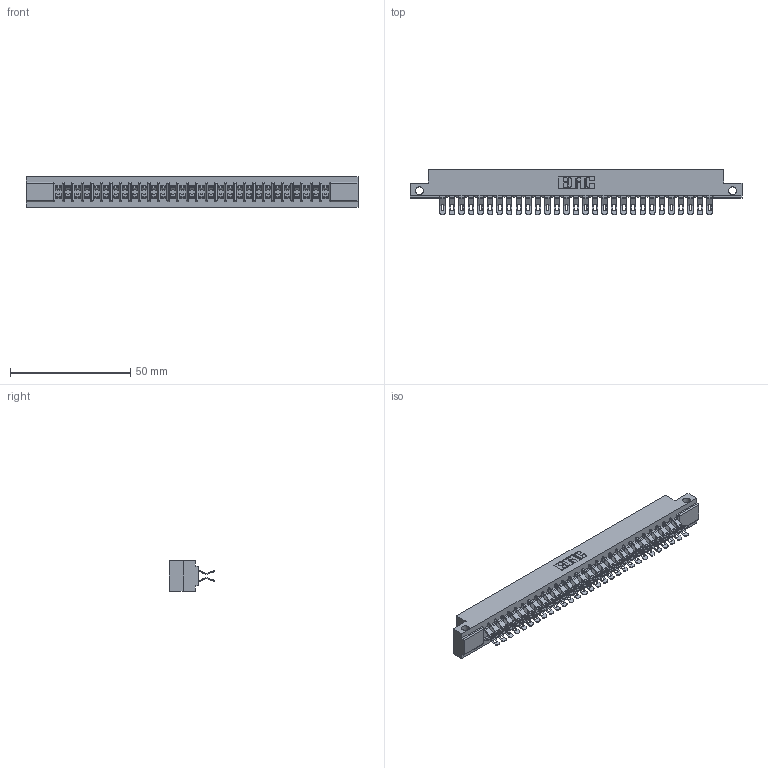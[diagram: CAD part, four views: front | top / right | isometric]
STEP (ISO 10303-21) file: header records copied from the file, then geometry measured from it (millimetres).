
FILE_DESCRIPTION (( 'STEP AP203' ), '1' );
FILE_NAME ('357-058-555-212.STEP', '2019-09-19T05:32:24', ( '' ), ( '' ), 'SwSTEP 2.0', 'SolidWorks 2016', '' );
FILE_SCHEMA (( 'CONFIG_CONTROL_DESIGN' ));
Length unit declared in the file: inch
Products named in the file (3): 357-058-555-212; 307-290-001_555; 307 Part_.128 Dia Side Mounting Holes
Assembly tree (59 placements, depth 2):
  357-058-555-212
    307 Part_.128 Dia Side Mounting Holes
    307-290-001_555  x58
Bounding box: 137.92 x 18.75 x 12.7 mm (x, y, z)
Volume: 14604.9 mm3; surface area: 18552.2 mm2
Topology: 59 solids, 59 shells, 3686 faces, 10821 edges, 7054 vertices
Faces by surface type: plane 2042, cylinder 1584, sphere 60
Entity records: 27931 total; most frequent: CARTESIAN_POINT 4577, ORIENTED_EDGE 4536, DIRECTION 4496, EDGE_CURVE 2268, LINE 1722, VECTOR 1722, VERTEX_POINT 1468, AXIS2_PLACEMENT_3D 1387
